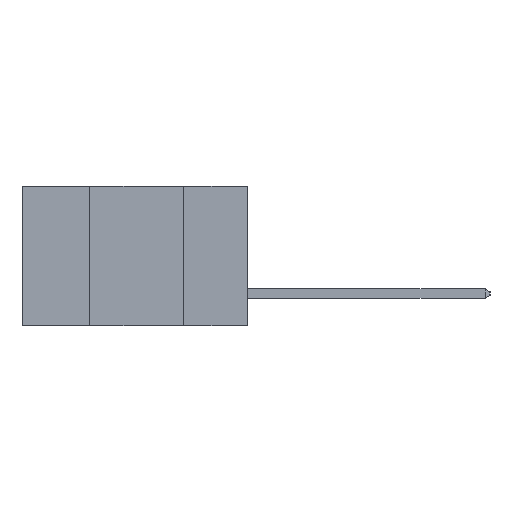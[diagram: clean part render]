
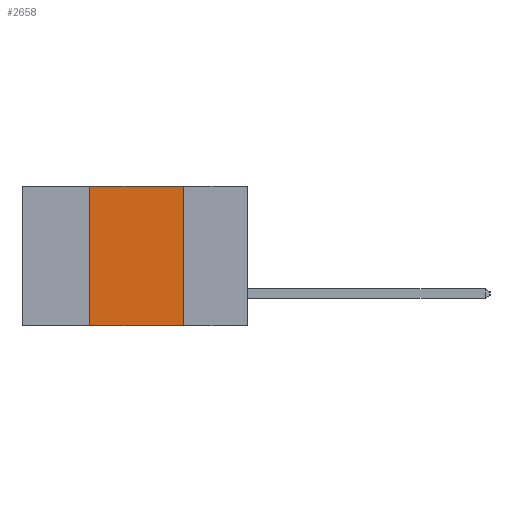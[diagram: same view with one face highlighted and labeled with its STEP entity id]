
A CAD part, left-side view. The second image highlights one B-rep face of the part: STEP entity #2658.
In plain terms, the highlighted planar face has unit normal (-1, 0, 0).
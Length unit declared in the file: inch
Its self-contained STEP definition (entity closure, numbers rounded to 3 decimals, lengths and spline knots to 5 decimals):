
#190 = PLANE ( 'NONE',  #3373 ) ;
#304 = ORIENTED_EDGE ( 'NONE', *, *, #6669, .F. ) ;
#638 = VECTOR ( 'NONE', #12922, 39.37008 ) ;
#764 = EDGE_LOOP ( 'NONE', ( #304, #1717, #11162, #6895 ) ) ;
#843 = CARTESIAN_POINT ( 'NONE',  ( 0., 0.17, 0. ) ) ;
#1462 = LINE ( 'NONE', #4095, #3877 ) ;
#1717 = ORIENTED_EDGE ( 'NONE', *, *, #10347, .F. ) ;
#2658 = ADVANCED_FACE ( 'NONE', ( #2662 ), #190, .F. ) ;
#2662 = FACE_OUTER_BOUND ( 'NONE', #764, .T. ) ;
#2796 = LINE ( 'NONE', #12978, #7971 ) ;
#3245 = CARTESIAN_POINT ( 'NONE',  ( 0., 0.42, -0.37 ) ) ;
#3373 = AXIS2_PLACEMENT_3D ( 'NONE', #5091, #4068, #8169 ) ;
#3737 = LINE ( 'NONE', #9192, #8250 ) ;
#3877 = VECTOR ( 'NONE', #4428, 39.37008 ) ;
#4026 = VERTEX_POINT ( 'NONE', #11316 ) ;
#4068 = DIRECTION ( 'NONE',  ( 1., 0., 0. ) ) ;
#4095 = CARTESIAN_POINT ( 'NONE',  ( 0., 0.17, -0.37 ) ) ;
#4428 = DIRECTION ( 'NONE',  ( 0., 0., -1. ) ) ;
#5091 = CARTESIAN_POINT ( 'NONE',  ( 0., 0.6, 0. ) ) ;
#5102 = CARTESIAN_POINT ( 'NONE',  ( 0., 0.42, 0. ) ) ;
#6110 = EDGE_CURVE ( 'NONE', #11977, #4026, #3737, .T. ) ;
#6618 = VERTEX_POINT ( 'NONE', #5102 ) ;
#6669 = EDGE_CURVE ( 'NONE', #7025, #4026, #1462, .T. ) ;
#6895 = ORIENTED_EDGE ( 'NONE', *, *, #6110, .T. ) ;
#7025 = VERTEX_POINT ( 'NONE', #843 ) ;
#7829 = CARTESIAN_POINT ( 'NONE',  ( 0., 0.42, -0.37 ) ) ;
#7884 = DIRECTION ( 'NONE',  ( 0., -1., 0. ) ) ;
#7971 = VECTOR ( 'NONE', #7884, 39.37008 ) ;
#8169 = DIRECTION ( 'NONE',  ( 0., 0., -1. ) ) ;
#8250 = VECTOR ( 'NONE', #9091, 39.37008 ) ;
#8882 = LINE ( 'NONE', #7829, #638 ) ;
#9091 = DIRECTION ( 'NONE',  ( 0., -1., 0. ) ) ;
#9192 = CARTESIAN_POINT ( 'NONE',  ( 0., 0.6, -0.37 ) ) ;
#10347 = EDGE_CURVE ( 'NONE', #6618, #7025, #2796, .T. ) ;
#11162 = ORIENTED_EDGE ( 'NONE', *, *, #12767, .F. ) ;
#11316 = CARTESIAN_POINT ( 'NONE',  ( 0., 0.17, -0.37 ) ) ;
#11977 = VERTEX_POINT ( 'NONE', #3245 ) ;
#12767 = EDGE_CURVE ( 'NONE', #11977, #6618, #8882, .T. ) ;
#12922 = DIRECTION ( 'NONE',  ( 0., 0., 1. ) ) ;
#12978 = CARTESIAN_POINT ( 'NONE',  ( 0., 0.6, 0. ) ) ;
